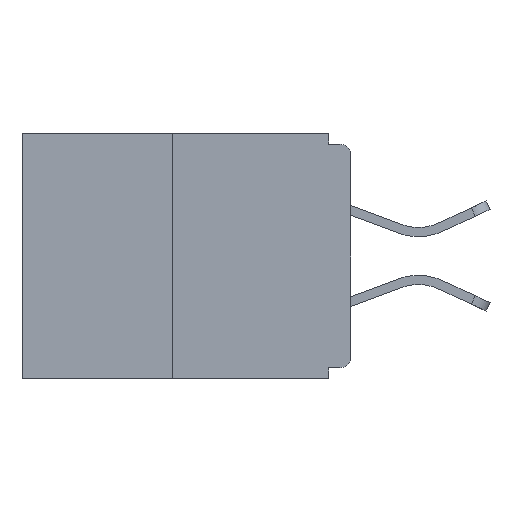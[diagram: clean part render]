
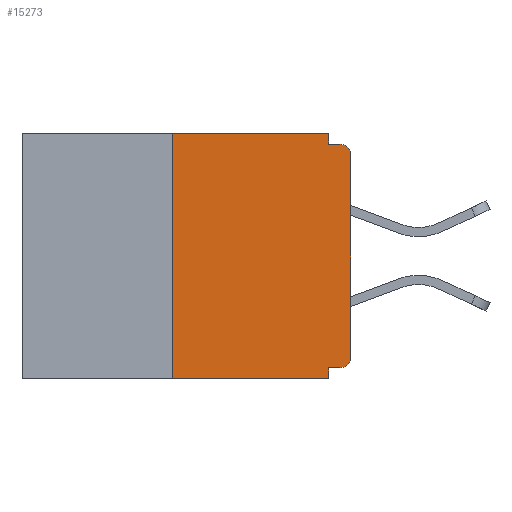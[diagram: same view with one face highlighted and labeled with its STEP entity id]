
A CAD part, left-side view. The second image highlights one B-rep face of the part: STEP entity #15273.
In plain terms, the highlighted planar face has unit normal (-1, 0, 0).
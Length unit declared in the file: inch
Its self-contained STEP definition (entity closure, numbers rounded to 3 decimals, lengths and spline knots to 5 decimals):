
#657 = DIRECTION ( 'NONE',  ( -1., 0., 0. ) ) ;
#831 = DIRECTION ( 'NONE',  ( 0., 0., -1. ) ) ;
#979 = EDGE_CURVE ( 'NONE', #16448, #3709, #7795, .T. ) ;
#984 = LINE ( 'NONE', #5800, #1382 ) ;
#1233 = DIRECTION ( 'NONE',  ( 0., 0., -1. ) ) ;
#1382 = VECTOR ( 'NONE', #1940, 39.37008 ) ;
#1573 = LINE ( 'NONE', #1744, #3033 ) ;
#1582 = CARTESIAN_POINT ( 'NONE',  ( 0., 0.031, -0.343 ) ) ;
#1744 = CARTESIAN_POINT ( 'NONE',  ( 0., 0., 0. ) ) ;
#1888 = EDGE_LOOP ( 'NONE', ( #13168, #4037, #17266, #3939, #10221, #4815, #5732, #15606, #2601, #7641 ) ) ;
#1940 = DIRECTION ( 'NONE',  ( 0., 0., 1. ) ) ;
#2039 = DIRECTION ( 'NONE',  ( 0., 1., 0. ) ) ;
#2285 = CARTESIAN_POINT ( 'NONE',  ( 0., 0.031, -0.343 ) ) ;
#2305 = CARTESIAN_POINT ( 'NONE',  ( 0., 0.031, -0.015 ) ) ;
#2314 = VERTEX_POINT ( 'NONE', #14422 ) ;
#2601 = ORIENTED_EDGE ( 'NONE', *, *, #979, .F. ) ;
#3033 = VECTOR ( 'NONE', #16407, 39.37008 ) ;
#3709 = VERTEX_POINT ( 'NONE', #9125 ) ;
#3927 = LINE ( 'NONE', #2285, #6247 ) ;
#3939 = ORIENTED_EDGE ( 'NONE', *, *, #17081, .F. ) ;
#3960 = VECTOR ( 'NONE', #2039, 39.37008 ) ;
#4037 = ORIENTED_EDGE ( 'NONE', *, *, #12416, .F. ) ;
#4331 = AXIS2_PLACEMENT_3D ( 'NONE', #7369, #657, #6022 ) ;
#4392 = PLANE ( 'NONE',  #10757 ) ;
#4815 = ORIENTED_EDGE ( 'NONE', *, *, #10026, .T. ) ;
#4831 = CARTESIAN_POINT ( 'NONE',  ( 0., 0.46, 0. ) ) ;
#4901 = CARTESIAN_POINT ( 'NONE',  ( 0., 0.015, -0.03 ) ) ;
#5161 = AXIS2_PLACEMENT_3D ( 'NONE', #4901, #11566, #831 ) ;
#5239 = CARTESIAN_POINT ( 'NONE',  ( 0., 0., -0.313 ) ) ;
#5732 = ORIENTED_EDGE ( 'NONE', *, *, #10436, .T. ) ;
#5800 = CARTESIAN_POINT ( 'NONE',  ( 0., 0.25, 0. ) ) ;
#6022 = DIRECTION ( 'NONE',  ( 0., 0., -1. ) ) ;
#6247 = VECTOR ( 'NONE', #1233, 39.37008 ) ;
#6505 = LINE ( 'NONE', #7160, #12572 ) ;
#6733 = FACE_OUTER_BOUND ( 'NONE', #1888, .T. ) ;
#6878 = CARTESIAN_POINT ( 'NONE',  ( 0., 0.031, 0. ) ) ;
#7001 = DIRECTION ( 'NONE',  ( 0., 0., -1. ) ) ;
#7160 = CARTESIAN_POINT ( 'NONE',  ( 0., 0.46, -0.343 ) ) ;
#7369 = CARTESIAN_POINT ( 'NONE',  ( 0., 0.015, -0.313 ) ) ;
#7641 = ORIENTED_EDGE ( 'NONE', *, *, #14615, .F. ) ;
#7795 = LINE ( 'NONE', #9355, #17177 ) ;
#7829 = VERTEX_POINT ( 'NONE', #9955 ) ;
#7845 = EDGE_CURVE ( 'NONE', #9365, #7829, #10898, .T. ) ;
#7921 = VERTEX_POINT ( 'NONE', #8549 ) ;
#8212 = DIRECTION ( 'NONE',  ( 0., -1., 0. ) ) ;
#8549 = CARTESIAN_POINT ( 'NONE',  ( 0., 0., -0.03 ) ) ;
#8951 = VECTOR ( 'NONE', #17038, 39.37008 ) ;
#9125 = CARTESIAN_POINT ( 'NONE',  ( 0., 0.015, -0.015 ) ) ;
#9281 = VERTEX_POINT ( 'NONE', #16680 ) ;
#9355 = CARTESIAN_POINT ( 'NONE',  ( 0., 0., -0.015 ) ) ;
#9365 = VERTEX_POINT ( 'NONE', #10222 ) ;
#9955 = CARTESIAN_POINT ( 'NONE',  ( 0., 0.031, -0.328 ) ) ;
#10026 = EDGE_CURVE ( 'NONE', #9365, #15547, #16212, .T. ) ;
#10135 = LINE ( 'NONE', #6878, #10550 ) ;
#10154 = EDGE_CURVE ( 'NONE', #9281, #13845, #15998, .T. ) ;
#10221 = ORIENTED_EDGE ( 'NONE', *, *, #7845, .F. ) ;
#10222 = CARTESIAN_POINT ( 'NONE',  ( 0., 0.015, -0.328 ) ) ;
#10436 = EDGE_CURVE ( 'NONE', #15547, #7921, #1573, .T. ) ;
#10550 = VECTOR ( 'NONE', #7001, 39.37008 ) ;
#10658 = EDGE_CURVE ( 'NONE', #7921, #3709, #14331, .T. ) ;
#10757 = AXIS2_PLACEMENT_3D ( 'NONE', #12353, #15034, #13755 ) ;
#10898 = LINE ( 'NONE', #13962, #3960 ) ;
#11566 = DIRECTION ( 'NONE',  ( -1., 0., 0. ) ) ;
#11934 = CARTESIAN_POINT ( 'NONE',  ( 0., 0.031, 0. ) ) ;
#12224 = DIRECTION ( 'NONE',  ( 0., -1., 0. ) ) ;
#12353 = CARTESIAN_POINT ( 'NONE',  ( 0., 0.46, 0. ) ) ;
#12416 = EDGE_CURVE ( 'NONE', #2314, #9281, #984, .T. ) ;
#12572 = VECTOR ( 'NONE', #12224, 39.37008 ) ;
#13168 = ORIENTED_EDGE ( 'NONE', *, *, #10154, .F. ) ;
#13755 = DIRECTION ( 'NONE',  ( 0., 0., -1. ) ) ;
#13845 = VERTEX_POINT ( 'NONE', #11934 ) ;
#13962 = CARTESIAN_POINT ( 'NONE',  ( 0., 0., -0.328 ) ) ;
#14331 = CIRCLE ( 'NONE', #5161, 0.015 ) ;
#14422 = CARTESIAN_POINT ( 'NONE',  ( 0., 0.25, -0.343 ) ) ;
#14615 = EDGE_CURVE ( 'NONE', #13845, #16448, #10135, .T. ) ;
#15034 = DIRECTION ( 'NONE',  ( 1., 0., 0. ) ) ;
#15273 = ADVANCED_FACE ( 'NONE', ( #6733 ), #4392, .F. ) ;
#15547 = VERTEX_POINT ( 'NONE', #5239 ) ;
#15606 = ORIENTED_EDGE ( 'NONE', *, *, #10658, .T. ) ;
#15852 = VERTEX_POINT ( 'NONE', #1582 ) ;
#15998 = LINE ( 'NONE', #4831, #8951 ) ;
#16172 = EDGE_CURVE ( 'NONE', #2314, #15852, #6505, .T. ) ;
#16212 = CIRCLE ( 'NONE', #4331, 0.015 ) ;
#16407 = DIRECTION ( 'NONE',  ( 0., 0., 1. ) ) ;
#16448 = VERTEX_POINT ( 'NONE', #2305 ) ;
#16680 = CARTESIAN_POINT ( 'NONE',  ( 0., 0.25, 0. ) ) ;
#17038 = DIRECTION ( 'NONE',  ( 0., -1., 0. ) ) ;
#17081 = EDGE_CURVE ( 'NONE', #7829, #15852, #3927, .T. ) ;
#17177 = VECTOR ( 'NONE', #8212, 39.37008 ) ;
#17266 = ORIENTED_EDGE ( 'NONE', *, *, #16172, .T. ) ;
